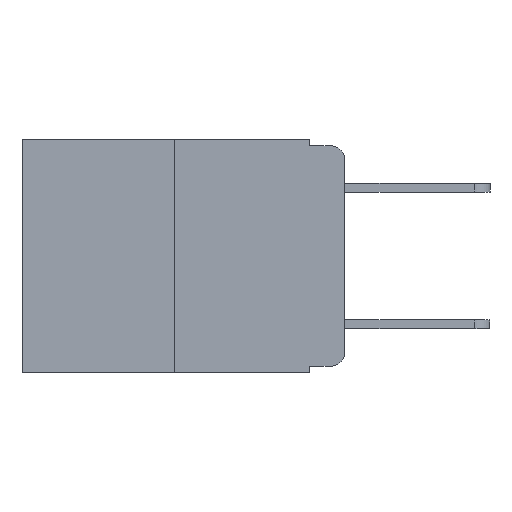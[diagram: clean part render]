
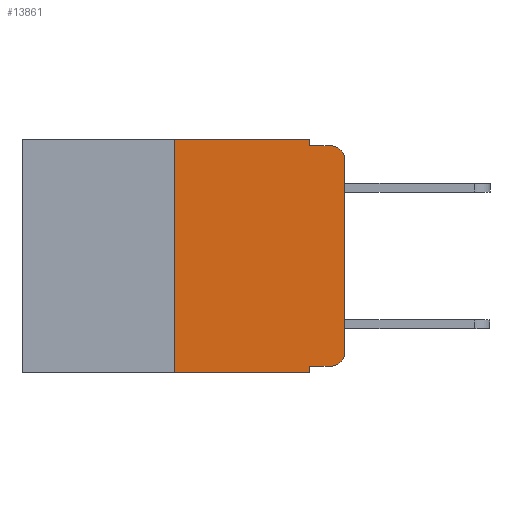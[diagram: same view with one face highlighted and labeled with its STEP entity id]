
A CAD part, left-side view. The second image highlights one B-rep face of the part: STEP entity #13861.
In plain terms, the highlighted planar face has unit normal (-1, 0, 0).
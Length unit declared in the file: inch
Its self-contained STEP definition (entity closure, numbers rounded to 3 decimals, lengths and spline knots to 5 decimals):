
#258 = ORIENTED_EDGE ( 'NONE', *, *, #1916, .T. ) ;
#431 = VECTOR ( 'NONE', #6592, 39.37008 ) ;
#911 = VERTEX_POINT ( 'NONE', #3838 ) ;
#1410 = ORIENTED_EDGE ( 'NONE', *, *, #4235, .F. ) ;
#1429 = VECTOR ( 'NONE', #4739, 39.37008 ) ;
#1557 = CARTESIAN_POINT ( 'NONE',  ( 0., 0.051, -0.333 ) ) ;
#1796 = DIRECTION ( 'NONE',  ( 0., -1., 0. ) ) ;
#1801 = VECTOR ( 'NONE', #4505, 39.37008 ) ;
#1916 = EDGE_CURVE ( 'NONE', #911, #9990, #6046, .T. ) ;
#2659 = EDGE_CURVE ( 'NONE', #9006, #12305, #15385, .T. ) ;
#2688 = VECTOR ( 'NONE', #5974, 39.37008 ) ;
#3113 = EDGE_CURVE ( 'NONE', #6711, #9990, #8015, .T. ) ;
#3229 = EDGE_CURVE ( 'NONE', #4690, #6711, #13367, .T. ) ;
#3243 = AXIS2_PLACEMENT_3D ( 'NONE', #13192, #5185, #14518 ) ;
#3339 = ORIENTED_EDGE ( 'NONE', *, *, #8984, .F. ) ;
#3678 = DIRECTION ( 'NONE',  ( 1., 0., 0. ) ) ;
#3681 = AXIS2_PLACEMENT_3D ( 'NONE', #7603, #3678, #13055 ) ;
#3838 = CARTESIAN_POINT ( 'NONE',  ( 0., 0., -0.03 ) ) ;
#3903 = EDGE_LOOP ( 'NONE', ( #16072, #258, #7861, #15427, #3339, #1410, #14446, #8093, #5462, #3978 ) ) ;
#3978 = ORIENTED_EDGE ( 'NONE', *, *, #2659, .T. ) ;
#4039 = CARTESIAN_POINT ( 'NONE',  ( 0., 0.051, 0. ) ) ;
#4235 = EDGE_CURVE ( 'NONE', #11475, #14741, #14748, .T. ) ;
#4453 = CARTESIAN_POINT ( 'NONE',  ( 0., 0.051, -0.01 ) ) ;
#4505 = DIRECTION ( 'NONE',  ( 0., -1., 0. ) ) ;
#4623 = CARTESIAN_POINT ( 'NONE',  ( 0., 0.051, 0. ) ) ;
#4670 = EDGE_CURVE ( 'NONE', #9566, #12591, #13512, .T. ) ;
#4690 = VERTEX_POINT ( 'NONE', #4039 ) ;
#4739 = DIRECTION ( 'NONE',  ( 0., -1., 0. ) ) ;
#4970 = CARTESIAN_POINT ( 'NONE',  ( 0., 0.473, 0. ) ) ;
#5048 = LINE ( 'NONE', #10011, #1429 ) ;
#5074 = CARTESIAN_POINT ( 'NONE',  ( 0., 0., -0.313 ) ) ;
#5185 = DIRECTION ( 'NONE',  ( -1., 0., 0. ) ) ;
#5462 = ORIENTED_EDGE ( 'NONE', *, *, #7946, .T. ) ;
#5708 = CARTESIAN_POINT ( 'NONE',  ( 0., 0.051, -0.343 ) ) ;
#5888 = CARTESIAN_POINT ( 'NONE',  ( 0., 0.25, 0. ) ) ;
#5890 = VECTOR ( 'NONE', #11633, 39.37008 ) ;
#5974 = DIRECTION ( 'NONE',  ( 0., 0., -1. ) ) ;
#6046 = CIRCLE ( 'NONE', #12845, 0.02 ) ;
#6365 = CARTESIAN_POINT ( 'NONE',  ( 0., 0.02, -0.333 ) ) ;
#6534 = CARTESIAN_POINT ( 'NONE',  ( 0., 0.25, 0. ) ) ;
#6592 = DIRECTION ( 'NONE',  ( 0., 0., 1. ) ) ;
#6691 = CARTESIAN_POINT ( 'NONE',  ( 0., 0.051, 0. ) ) ;
#6704 = DIRECTION ( 'NONE',  ( -1., 0., 0. ) ) ;
#6711 = VERTEX_POINT ( 'NONE', #17078 ) ;
#7015 = VECTOR ( 'NONE', #7178, 39.37008 ) ;
#7178 = DIRECTION ( 'NONE',  ( 0., 0., 1. ) ) ;
#7431 = VECTOR ( 'NONE', #1796, 39.37008 ) ;
#7603 = CARTESIAN_POINT ( 'NONE',  ( 0., 0.473, 0. ) ) ;
#7861 = ORIENTED_EDGE ( 'NONE', *, *, #3113, .F. ) ;
#7946 = EDGE_CURVE ( 'NONE', #9566, #9006, #5048, .T. ) ;
#8015 = LINE ( 'NONE', #4453, #7431 ) ;
#8093 = ORIENTED_EDGE ( 'NONE', *, *, #4670, .F. ) ;
#8918 = PLANE ( 'NONE',  #3681 ) ;
#8984 = EDGE_CURVE ( 'NONE', #14741, #4690, #10249, .T. ) ;
#9006 = VERTEX_POINT ( 'NONE', #6365 ) ;
#9566 = VERTEX_POINT ( 'NONE', #1557 ) ;
#9990 = VERTEX_POINT ( 'NONE', #16985 ) ;
#10011 = CARTESIAN_POINT ( 'NONE',  ( 0., 0.051, -0.333 ) ) ;
#10249 = LINE ( 'NONE', #4970, #5890 ) ;
#11475 = VERTEX_POINT ( 'NONE', #14443 ) ;
#11633 = DIRECTION ( 'NONE',  ( 0., -1., 0. ) ) ;
#12305 = VERTEX_POINT ( 'NONE', #5074 ) ;
#12486 = LINE ( 'NONE', #12498, #1801 ) ;
#12498 = CARTESIAN_POINT ( 'NONE',  ( 0., 0.473, -0.343 ) ) ;
#12591 = VERTEX_POINT ( 'NONE', #5708 ) ;
#12845 = AXIS2_PLACEMENT_3D ( 'NONE', #14688, #6704, #16041 ) ;
#13055 = DIRECTION ( 'NONE',  ( 0., 0., -1. ) ) ;
#13085 = VECTOR ( 'NONE', #13366, 39.37008 ) ;
#13192 = CARTESIAN_POINT ( 'NONE',  ( 0., 0.02, -0.313 ) ) ;
#13366 = DIRECTION ( 'NONE',  ( 0., 0., -1. ) ) ;
#13367 = LINE ( 'NONE', #4623, #2688 ) ;
#13512 = LINE ( 'NONE', #6691, #13085 ) ;
#13861 = ADVANCED_FACE ( 'NONE', ( #16376 ), #8918, .F. ) ;
#13907 = CARTESIAN_POINT ( 'NONE',  ( 0., 0., 0. ) ) ;
#14443 = CARTESIAN_POINT ( 'NONE',  ( 0., 0.25, -0.343 ) ) ;
#14446 = ORIENTED_EDGE ( 'NONE', *, *, #15882, .T. ) ;
#14518 = DIRECTION ( 'NONE',  ( 0., 0., -1. ) ) ;
#14550 = LINE ( 'NONE', #13907, #7015 ) ;
#14688 = CARTESIAN_POINT ( 'NONE',  ( 0., 0.02, -0.03 ) ) ;
#14741 = VERTEX_POINT ( 'NONE', #5888 ) ;
#14748 = LINE ( 'NONE', #6534, #431 ) ;
#15385 = CIRCLE ( 'NONE', #3243, 0.02 ) ;
#15427 = ORIENTED_EDGE ( 'NONE', *, *, #3229, .F. ) ;
#15882 = EDGE_CURVE ( 'NONE', #11475, #12591, #12486, .T. ) ;
#16041 = DIRECTION ( 'NONE',  ( 0., 0., -1. ) ) ;
#16072 = ORIENTED_EDGE ( 'NONE', *, *, #16397, .T. ) ;
#16376 = FACE_OUTER_BOUND ( 'NONE', #3903, .T. ) ;
#16397 = EDGE_CURVE ( 'NONE', #12305, #911, #14550, .T. ) ;
#16985 = CARTESIAN_POINT ( 'NONE',  ( 0., 0.02, -0.01 ) ) ;
#17078 = CARTESIAN_POINT ( 'NONE',  ( 0., 0.051, -0.01 ) ) ;
